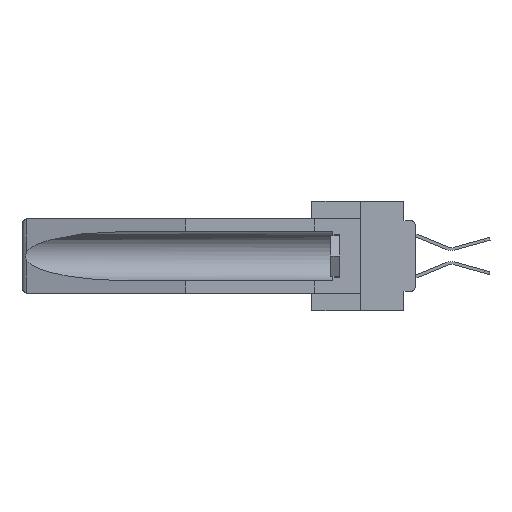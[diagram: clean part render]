
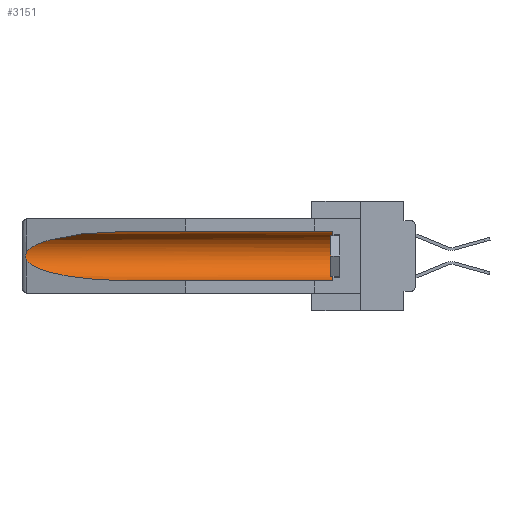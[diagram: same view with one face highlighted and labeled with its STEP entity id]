
A CAD part, left-side view. The second image highlights one B-rep face of the part: STEP entity #3151.
In plain terms, the highlighted cylindrical face has radius 2.857 mm (diameter 5.715 mm), a partial arc.
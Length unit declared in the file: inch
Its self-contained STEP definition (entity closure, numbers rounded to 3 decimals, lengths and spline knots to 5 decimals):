
#1775 = CARTESIAN_POINT ( 'NONE',  ( 0.2673, 1.5327, -0.16383 ) ) ;
#2890 = CARTESIAN_POINT ( 'NONE',  ( 0.25451, 1.48313, -0.24835 ) ) ;
#3151 = ADVANCED_FACE ( 'NONE', ( #26223 ), #17886, .F. ) ;
#3808 = ORIENTED_EDGE ( 'NONE', *, *, #25427, .T. ) ;
#3981 = AXIS2_PLACEMENT_3D ( 'NONE', #27678, #30013, #12197 ) ;
#4447 = CARTESIAN_POINT ( 'NONE',  ( 0.26597, 1.52961, -0.15275 ) ) ;
#5000 = CARTESIAN_POINT ( 'NONE',  ( 0.155, 1.07973, -0.284 ) ) ;
#6099 = EDGE_CURVE ( 'NONE', #13937, #32074, #23067, .T. ) ;
#6130 = VERTEX_POINT ( 'NONE', #5000 ) ;
#6785 = CARTESIAN_POINT ( 'NONE',  ( 0.26537, 1.52718, -0.14972 ) ) ;
#7389 = CARTESIAN_POINT ( 'NONE',  ( 0.155, 0.126, -0.1715 ) ) ;
#7678 = VERTEX_POINT ( 'NONE', #13059 ) ;
#8238 = EDGE_CURVE ( 'NONE', #15493, #6130, #25520, .T. ) ;
#8462 = CARTESIAN_POINT ( 'NONE',  ( 0.155, -0.30754, -0.284 ) ) ;
#9593 = CARTESIAN_POINT ( 'NONE',  ( 0.26654, 1.53092, -0.15636 ) ) ;
#9932 = ORIENTED_EDGE ( 'NONE', *, *, #8238, .T. ) ;
#12197 = DIRECTION ( 'NONE',  ( 0., 0., 1. ) ) ;
#13059 = CARTESIAN_POINT ( 'NONE',  ( 0.155, 0.126, -0.059 ) ) ;
#13937 = VERTEX_POINT ( 'NONE', #17456 ) ;
#14054 = CIRCLE ( 'NONE', #30442, 0.1125 ) ;
#14433 = VECTOR ( 'NONE', #17594, 39.37008 ) ;
#14587 = CARTESIAN_POINT ( 'NONE',  ( 0.26655, 1.53094, -0.18657 ) ) ;
#15093 = DIRECTION ( 'NONE',  ( 0., 0., 1. ) ) ;
#15493 = VERTEX_POINT ( 'NONE', #16324 ) ;
#16189 = ORIENTED_EDGE ( 'NONE', *, *, #25008, .F. ) ;
#16324 = CARTESIAN_POINT ( 'NONE',  ( 0.26537, 1.52718, -0.19328 ) ) ;
#16854 = VERTEX_POINT ( 'NONE', #27237 ) ;
#16938 = CARTESIAN_POINT ( 'NONE',  ( 0.155, 1.07973, -0.059 ) ) ;
#17364 = CARTESIAN_POINT ( 'NONE',  ( 0.26537, 1.52718, -0.14972 ) ) ;
#17456 = CARTESIAN_POINT ( 'NONE',  ( 0.155, 1.07973, -0.059 ) ) ;
#17594 = DIRECTION ( 'NONE',  ( 0., 1., 0. ) ) ;
#17886 = CYLINDRICAL_SURFACE ( 'NONE', #3981, 0.1125 ) ;
#19503 = CARTESIAN_POINT ( 'NONE',  ( 0.21114, 1.30732, -0.059 ) ) ;
#20218 = B_SPLINE_CURVE_WITH_KNOTS ( 'NONE', 3,
 ( #24600, #4447, #9593, #1775, #29856, #22047, #24830, #14587, #24383, #29624 ),
 .UNSPECIFIED., .F., .F.,
 ( 4, 2, 2, 2, 4 ),
 ( 0., 0.00029, 0.00058, 0.00087, 0.00117 ),
 .UNSPECIFIED. ) ;
#22047 = CARTESIAN_POINT ( 'NONE',  ( 0.2675, 1.53308, -0.17534 ) ) ;
#22248 = ORIENTED_EDGE ( 'NONE', *, *, #6099, .T. ) ;
#23067 =( BOUNDED_CURVE ( )  B_SPLINE_CURVE ( 3, ( #16938, #19503, #24471, #6785 ),
 .UNSPECIFIED., .F., .F. ) 
 B_SPLINE_CURVE_WITH_KNOTS ( ( 4, 4 ),
 ( 4.71239, 6.08839 ),
 .UNSPECIFIED. ) 
 CURVE ( )  GEOMETRIC_REPRESENTATION_ITEM ( )  RATIONAL_B_SPLINE_CURVE ( ( 1., 0.848, 0.848, 1. ) ) 
 REPRESENTATION_ITEM ( '' )  );
#23491 = CARTESIAN_POINT ( 'NONE',  ( 0.21114, 1.30732, -0.284 ) ) ;
#23602 = LINE ( 'NONE', #8462, #29570 ) ;
#24383 = CARTESIAN_POINT ( 'NONE',  ( 0.26597, 1.5296, -0.19026 ) ) ;
#24471 = CARTESIAN_POINT ( 'NONE',  ( 0.25451, 1.48313, -0.09465 ) ) ;
#24600 = CARTESIAN_POINT ( 'NONE',  ( 0.26537, 1.52718, -0.14972 ) ) ;
#24830 = CARTESIAN_POINT ( 'NONE',  ( 0.2673, 1.53269, -0.17917 ) ) ;
#25008 = EDGE_CURVE ( 'NONE', #16854, #6130, #23602, .T. ) ;
#25213 = DIRECTION ( 'NONE',  ( 0., -1., 0. ) ) ;
#25427 = EDGE_CURVE ( 'NONE', #7678, #13937, #28788, .T. ) ;
#25437 = ORIENTED_EDGE ( 'NONE', *, *, #30869, .T. ) ;
#25520 =( BOUNDED_CURVE ( )  B_SPLINE_CURVE ( 3, ( #28503, #2890, #23491, #31057 ),
 .UNSPECIFIED., .F., .F. ) 
 B_SPLINE_CURVE_WITH_KNOTS ( ( 4, 4 ),
 ( 0.1948, 1.5708 ),
 .UNSPECIFIED. ) 
 CURVE ( )  GEOMETRIC_REPRESENTATION_ITEM ( )  RATIONAL_B_SPLINE_CURVE ( ( 1., 0.848, 0.848, 1. ) ) 
 REPRESENTATION_ITEM ( '' )  );
#26223 = FACE_OUTER_BOUND ( 'NONE', #30092, .T. ) ;
#26564 = EDGE_CURVE ( 'NONE', #32074, #15493, #20218, .T. ) ;
#27237 = CARTESIAN_POINT ( 'NONE',  ( 0.155, 0.126, -0.284 ) ) ;
#27678 = CARTESIAN_POINT ( 'NONE',  ( 0.155, -0.30754, -0.1715 ) ) ;
#28503 = CARTESIAN_POINT ( 'NONE',  ( 0.26537, 1.52718, -0.19328 ) ) ;
#28622 = DIRECTION ( 'NONE',  ( 0., 1., 0. ) ) ;
#28788 = LINE ( 'NONE', #30710, #14433 ) ;
#29570 = VECTOR ( 'NONE', #28622, 39.37008 ) ;
#29624 = CARTESIAN_POINT ( 'NONE',  ( 0.26537, 1.52718, -0.19328 ) ) ;
#29856 = CARTESIAN_POINT ( 'NONE',  ( 0.2675, 1.53308, -0.16763 ) ) ;
#30013 = DIRECTION ( 'NONE',  ( 0., 1., 0. ) ) ;
#30092 = EDGE_LOOP ( 'NONE', ( #22248, #32936, #9932, #16189, #25437, #3808 ) ) ;
#30442 = AXIS2_PLACEMENT_3D ( 'NONE', #7389, #25213, #15093 ) ;
#30710 = CARTESIAN_POINT ( 'NONE',  ( 0.155, -0.30754, -0.059 ) ) ;
#30869 = EDGE_CURVE ( 'NONE', #16854, #7678, #14054, .T. ) ;
#31057 = CARTESIAN_POINT ( 'NONE',  ( 0.155, 1.07973, -0.284 ) ) ;
#32074 = VERTEX_POINT ( 'NONE', #17364 ) ;
#32936 = ORIENTED_EDGE ( 'NONE', *, *, #26564, .T. ) ;
